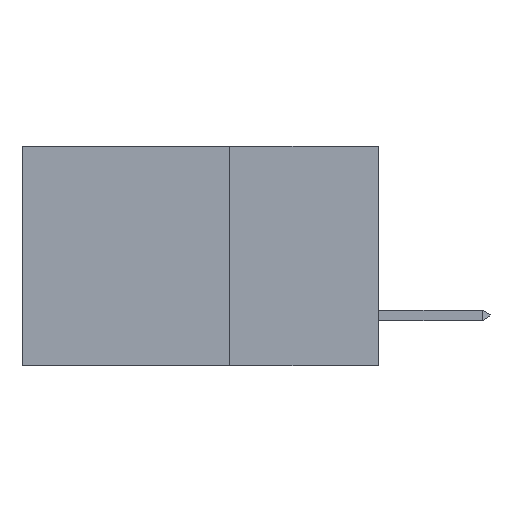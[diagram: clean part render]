
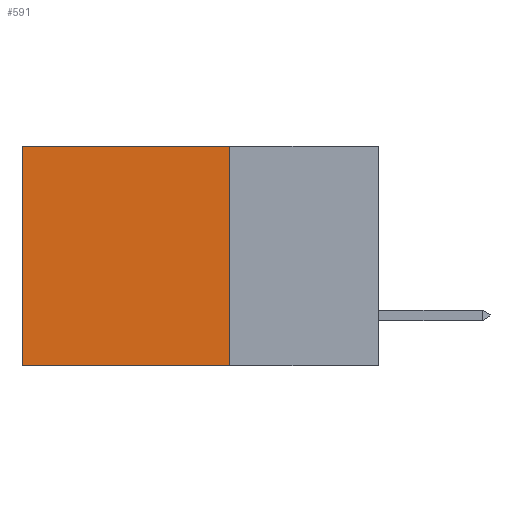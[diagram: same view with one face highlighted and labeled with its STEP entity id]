
A CAD part, left-side view. The second image highlights one B-rep face of the part: STEP entity #591.
In plain terms, the highlighted planar face has unit normal (-1, 0, 0).
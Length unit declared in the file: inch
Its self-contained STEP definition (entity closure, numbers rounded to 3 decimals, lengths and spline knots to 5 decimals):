
#554 = VERTEX_POINT ( 'NONE', #6179 ) ;
#591 = ADVANCED_FACE ( 'NONE', ( #5730 ), #12854, .F. ) ;
#956 = VERTEX_POINT ( 'NONE', #8776 ) ;
#1634 = ORIENTED_EDGE ( 'NONE', *, *, #3645, .F. ) ;
#1920 = ORIENTED_EDGE ( 'NONE', *, *, #12061, .F. ) ;
#1950 = DIRECTION ( 'NONE',  ( 0., 1., 0. ) ) ;
#2352 = CARTESIAN_POINT ( 'NONE',  ( 0.298, 0.25, 0. ) ) ;
#2450 = EDGE_LOOP ( 'NONE', ( #6051, #1920, #1634, #8724 ) ) ;
#2685 = VECTOR ( 'NONE', #18102, 39.37008 ) ;
#3645 = EDGE_CURVE ( 'NONE', #11932, #18185, #12985, .T. ) ;
#3704 = DIRECTION ( 'NONE',  ( 0., 1., 0. ) ) ;
#3860 = VECTOR ( 'NONE', #11241, 39.37008 ) ;
#4451 = DIRECTION ( 'NONE',  ( 1., 0., 0. ) ) ;
#5730 = FACE_OUTER_BOUND ( 'NONE', #2450, .T. ) ;
#6051 = ORIENTED_EDGE ( 'NONE', *, *, #9603, .T. ) ;
#6179 = CARTESIAN_POINT ( 'NONE',  ( 0.298, 0.6, -0.37 ) ) ;
#8043 = DIRECTION ( 'NONE',  ( 0., 0., -1. ) ) ;
#8062 = EDGE_CURVE ( 'NONE', #11932, #956, #22141, .T. ) ;
#8724 = ORIENTED_EDGE ( 'NONE', *, *, #8062, .T. ) ;
#8776 = CARTESIAN_POINT ( 'NONE',  ( 0.298, 0.6, 0. ) ) ;
#9603 = EDGE_CURVE ( 'NONE', #956, #554, #16879, .T. ) ;
#11241 = DIRECTION ( 'NONE',  ( 0., 0., -1. ) ) ;
#11525 = AXIS2_PLACEMENT_3D ( 'NONE', #18136, #4451, #8043 ) ;
#11932 = VERTEX_POINT ( 'NONE', #2352 ) ;
#12061 = EDGE_CURVE ( 'NONE', #18185, #554, #21567, .T. ) ;
#12807 = CARTESIAN_POINT ( 'NONE',  ( 0.298, 0.6, 0. ) ) ;
#12834 = CARTESIAN_POINT ( 'NONE',  ( 0.298, 0.25, 0. ) ) ;
#12854 = PLANE ( 'NONE',  #11525 ) ;
#12985 = LINE ( 'NONE', #12834, #3860 ) ;
#13607 = CARTESIAN_POINT ( 'NONE',  ( 0.298, 0.25, 0. ) ) ;
#13978 = CARTESIAN_POINT ( 'NONE',  ( 0.298, 0.25, -0.37 ) ) ;
#14943 = VECTOR ( 'NONE', #1950, 39.37008 ) ;
#16879 = LINE ( 'NONE', #12807, #2685 ) ;
#18102 = DIRECTION ( 'NONE',  ( 0., 0., -1. ) ) ;
#18136 = CARTESIAN_POINT ( 'NONE',  ( 0.298, 0.25, 0. ) ) ;
#18185 = VERTEX_POINT ( 'NONE', #21713 ) ;
#18934 = VECTOR ( 'NONE', #3704, 39.37008 ) ;
#21567 = LINE ( 'NONE', #13978, #18934 ) ;
#21713 = CARTESIAN_POINT ( 'NONE',  ( 0.298, 0.25, -0.37 ) ) ;
#22141 = LINE ( 'NONE', #13607, #14943 ) ;
